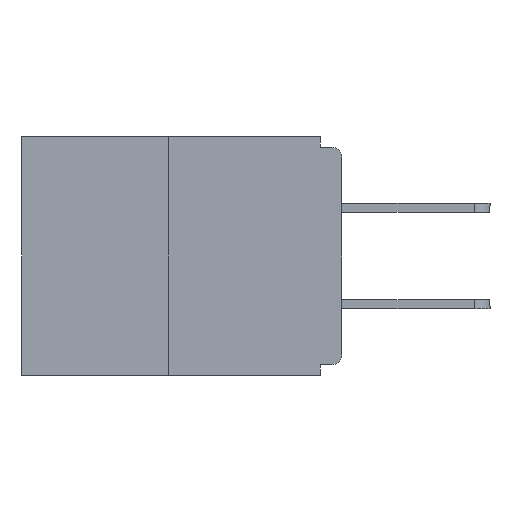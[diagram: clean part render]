
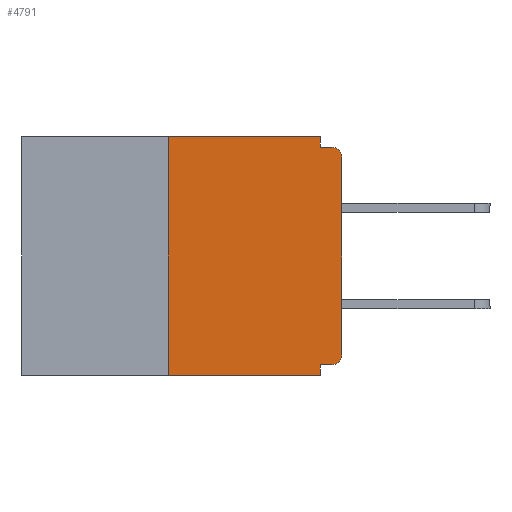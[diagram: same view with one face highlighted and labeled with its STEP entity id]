
A CAD part, left-side view. The second image highlights one B-rep face of the part: STEP entity #4791.
In plain terms, the highlighted planar face has unit normal (-1, 0, 0).
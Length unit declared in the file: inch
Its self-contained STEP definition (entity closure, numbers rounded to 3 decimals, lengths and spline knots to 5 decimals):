
#255 = CIRCLE ( 'NONE', #25604, 0.015 ) ;
#445 = FACE_OUTER_BOUND ( 'NONE', #24259, .T. ) ;
#1044 = ORIENTED_EDGE ( 'NONE', *, *, #8686, .F. ) ;
#1152 = VECTOR ( 'NONE', #13982, 39.37008 ) ;
#1272 = EDGE_CURVE ( 'NONE', #25983, #25745, #26940, .T. ) ;
#1342 = VERTEX_POINT ( 'NONE', #2614 ) ;
#1424 = VERTEX_POINT ( 'NONE', #11576 ) ;
#1837 = CARTESIAN_POINT ( 'NONE',  ( 0., 0., -0.015 ) ) ;
#2483 = CARTESIAN_POINT ( 'NONE',  ( 0., 0.46, -0.343 ) ) ;
#2614 = CARTESIAN_POINT ( 'NONE',  ( 0., 0., -0.313 ) ) ;
#3896 = LINE ( 'NONE', #15500, #5632 ) ;
#4093 = DIRECTION ( 'NONE',  ( 1., 0., 0. ) ) ;
#4111 = CARTESIAN_POINT ( 'NONE',  ( 0., 0.015, -0.03 ) ) ;
#4791 = ADVANCED_FACE ( 'NONE', ( #445 ), #28955, .F. ) ;
#5632 = VECTOR ( 'NONE', #13345, 39.37008 ) ;
#5934 = VERTEX_POINT ( 'NONE', #23683 ) ;
#7605 = LINE ( 'NONE', #15814, #25493 ) ;
#7660 = VECTOR ( 'NONE', #20616, 39.37008 ) ;
#8016 = VECTOR ( 'NONE', #9102, 39.37008 ) ;
#8063 = ORIENTED_EDGE ( 'NONE', *, *, #1272, .F. ) ;
#8670 = AXIS2_PLACEMENT_3D ( 'NONE', #4111, #13198, #20066 ) ;
#8686 = EDGE_CURVE ( 'NONE', #25480, #25983, #3896, .T. ) ;
#8996 = ORIENTED_EDGE ( 'NONE', *, *, #17694, .T. ) ;
#9102 = DIRECTION ( 'NONE',  ( 0., 1., 0. ) ) ;
#9310 = EDGE_CURVE ( 'NONE', #1342, #12398, #16430, .T. ) ;
#9389 = DIRECTION ( 'NONE',  ( 0., 0., -1. ) ) ;
#9491 = VERTEX_POINT ( 'NONE', #23949 ) ;
#9622 = CIRCLE ( 'NONE', #8670, 0.015 ) ;
#9639 = EDGE_CURVE ( 'NONE', #9491, #22765, #20626, .T. ) ;
#9772 = ORIENTED_EDGE ( 'NONE', *, *, #10850, .T. ) ;
#10074 = ORIENTED_EDGE ( 'NONE', *, *, #24595, .F. ) ;
#10850 = EDGE_CURVE ( 'NONE', #9491, #1342, #255, .T. ) ;
#11002 = CARTESIAN_POINT ( 'NONE',  ( 0., 0.031, -0.328 ) ) ;
#11404 = DIRECTION ( 'NONE',  ( 0., 0., 1. ) ) ;
#11576 = CARTESIAN_POINT ( 'NONE',  ( 0., 0.015, -0.015 ) ) ;
#11790 = DIRECTION ( 'NONE',  ( 0., 0., -1. ) ) ;
#12189 = VECTOR ( 'NONE', #11790, 39.37008 ) ;
#12398 = VERTEX_POINT ( 'NONE', #24521 ) ;
#13060 = CARTESIAN_POINT ( 'NONE',  ( 0., 0.031, -0.343 ) ) ;
#13198 = DIRECTION ( 'NONE',  ( -1., 0., 0. ) ) ;
#13345 = DIRECTION ( 'NONE',  ( 0., -1., 0. ) ) ;
#13463 = ORIENTED_EDGE ( 'NONE', *, *, #20387, .F. ) ;
#13982 = DIRECTION ( 'NONE',  ( 0., 0., -1. ) ) ;
#14084 = CARTESIAN_POINT ( 'NONE',  ( 0., 0.031, -0.343 ) ) ;
#15317 = CARTESIAN_POINT ( 'NONE',  ( 0., 0.031, -0.015 ) ) ;
#15500 = CARTESIAN_POINT ( 'NONE',  ( 0., 0.46, 0. ) ) ;
#15655 = ORIENTED_EDGE ( 'NONE', *, *, #18106, .T. ) ;
#15814 = CARTESIAN_POINT ( 'NONE',  ( 0., 0.25, 0. ) ) ;
#16430 = LINE ( 'NONE', #27464, #7660 ) ;
#16560 = ORIENTED_EDGE ( 'NONE', *, *, #23208, .F. ) ;
#16947 = LINE ( 'NONE', #1837, #26753 ) ;
#17001 = CARTESIAN_POINT ( 'NONE',  ( 0., 0.25, 0. ) ) ;
#17473 = DIRECTION ( 'NONE',  ( 0., -1., 0. ) ) ;
#17694 = EDGE_CURVE ( 'NONE', #12398, #1424, #9622, .T. ) ;
#17787 = CARTESIAN_POINT ( 'NONE',  ( 0., 0.46, 0. ) ) ;
#18106 = EDGE_CURVE ( 'NONE', #5934, #22565, #18611, .T. ) ;
#18162 = ORIENTED_EDGE ( 'NONE', *, *, #9310, .T. ) ;
#18281 = LINE ( 'NONE', #14084, #1152 ) ;
#18611 = LINE ( 'NONE', #2483, #20373 ) ;
#19018 = CARTESIAN_POINT ( 'NONE',  ( 0., 0.031, 0. ) ) ;
#20066 = DIRECTION ( 'NONE',  ( 0., 0., -1. ) ) ;
#20373 = VECTOR ( 'NONE', #20405, 39.37008 ) ;
#20387 = EDGE_CURVE ( 'NONE', #5934, #25480, #7605, .T. ) ;
#20405 = DIRECTION ( 'NONE',  ( 0., -1., 0. ) ) ;
#20616 = DIRECTION ( 'NONE',  ( 0., 0., 1. ) ) ;
#20626 = LINE ( 'NONE', #22546, #8016 ) ;
#20948 = DIRECTION ( 'NONE',  ( -1., 0., 0. ) ) ;
#22320 = DIRECTION ( 'NONE',  ( 0., 0., -1. ) ) ;
#22546 = CARTESIAN_POINT ( 'NONE',  ( 0., 0., -0.328 ) ) ;
#22565 = VERTEX_POINT ( 'NONE', #13060 ) ;
#22765 = VERTEX_POINT ( 'NONE', #11002 ) ;
#23208 = EDGE_CURVE ( 'NONE', #25745, #1424, #16947, .T. ) ;
#23683 = CARTESIAN_POINT ( 'NONE',  ( 0., 0.25, -0.343 ) ) ;
#23949 = CARTESIAN_POINT ( 'NONE',  ( 0., 0.015, -0.328 ) ) ;
#24259 = EDGE_LOOP ( 'NONE', ( #1044, #13463, #15655, #10074, #26325, #9772, #18162, #8996, #16560, #8063 ) ) ;
#24521 = CARTESIAN_POINT ( 'NONE',  ( 0., 0., -0.03 ) ) ;
#24595 = EDGE_CURVE ( 'NONE', #22765, #22565, #18281, .T. ) ;
#25124 = CARTESIAN_POINT ( 'NONE',  ( 0., 0.031, 0. ) ) ;
#25361 = CARTESIAN_POINT ( 'NONE',  ( 0., 0.015, -0.313 ) ) ;
#25480 = VERTEX_POINT ( 'NONE', #17001 ) ;
#25493 = VECTOR ( 'NONE', #11404, 39.37008 ) ;
#25567 = AXIS2_PLACEMENT_3D ( 'NONE', #17787, #4093, #22320 ) ;
#25604 = AXIS2_PLACEMENT_3D ( 'NONE', #25361, #20948, #9389 ) ;
#25745 = VERTEX_POINT ( 'NONE', #15317 ) ;
#25983 = VERTEX_POINT ( 'NONE', #19018 ) ;
#26325 = ORIENTED_EDGE ( 'NONE', *, *, #9639, .F. ) ;
#26753 = VECTOR ( 'NONE', #17473, 39.37008 ) ;
#26940 = LINE ( 'NONE', #25124, #12189 ) ;
#27464 = CARTESIAN_POINT ( 'NONE',  ( 0., 0., 0. ) ) ;
#28955 = PLANE ( 'NONE',  #25567 ) ;
